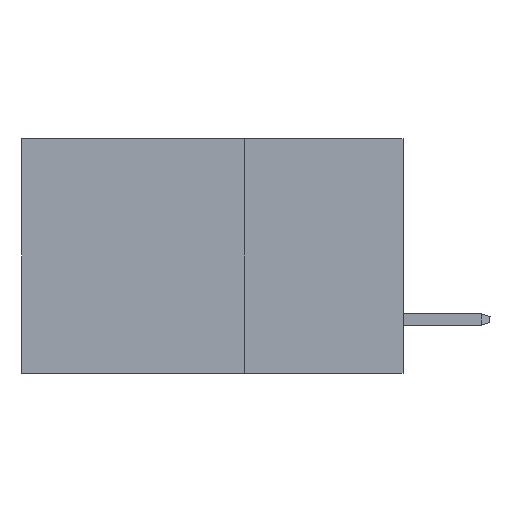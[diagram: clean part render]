
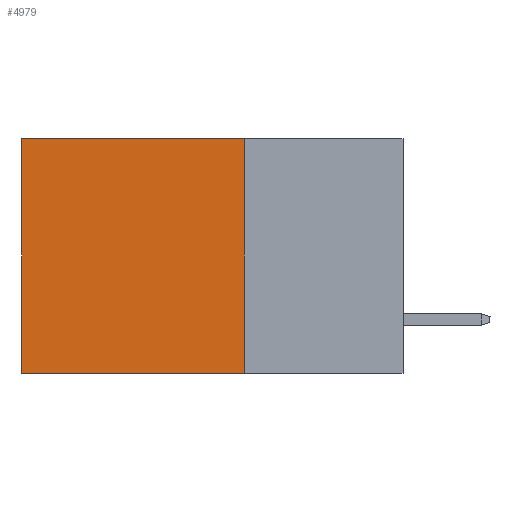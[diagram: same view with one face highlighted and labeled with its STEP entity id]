
A CAD part, left-side view. The second image highlights one B-rep face of the part: STEP entity #4979.
In plain terms, the highlighted planar face has unit normal (-1, 0, 0).
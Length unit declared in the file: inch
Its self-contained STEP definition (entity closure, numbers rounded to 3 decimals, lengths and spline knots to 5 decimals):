
#109 = VERTEX_POINT ( 'NONE', #10865 ) ;
#342 = ORIENTED_EDGE ( 'NONE', *, *, #12802, .T. ) ;
#1265 = CARTESIAN_POINT ( 'NONE',  ( 0.2875, 0.25, 0. ) ) ;
#1464 = CARTESIAN_POINT ( 'NONE',  ( 0.2875, 0.6, 0. ) ) ;
#2027 = ORIENTED_EDGE ( 'NONE', *, *, #6396, .F. ) ;
#2131 = VECTOR ( 'NONE', #9595, 39.37008 ) ;
#2871 = DIRECTION ( 'NONE',  ( 1., 0., 0. ) ) ;
#3625 = VERTEX_POINT ( 'NONE', #3956 ) ;
#3956 = CARTESIAN_POINT ( 'NONE',  ( 0.2875, 0.25, 0. ) ) ;
#4029 = FACE_OUTER_BOUND ( 'NONE', #9626, .T. ) ;
#4313 = VERTEX_POINT ( 'NONE', #4517 ) ;
#4517 = CARTESIAN_POINT ( 'NONE',  ( 0.2875, 0.6, 0. ) ) ;
#4924 = CARTESIAN_POINT ( 'NONE',  ( 0.2875, 0.25, -0.37 ) ) ;
#4979 = ADVANCED_FACE ( 'NONE', ( #4029 ), #5988, .F. ) ;
#5329 = EDGE_CURVE ( 'NONE', #4313, #109, #6518, .T. ) ;
#5395 = DIRECTION ( 'NONE',  ( 0., 0., -1. ) ) ;
#5525 = DIRECTION ( 'NONE',  ( 0., 0., -1. ) ) ;
#5896 = ORIENTED_EDGE ( 'NONE', *, *, #7676, .F. ) ;
#5988 = PLANE ( 'NONE',  #11218 ) ;
#6044 = DIRECTION ( 'NONE',  ( 0., 1., 0. ) ) ;
#6396 = EDGE_CURVE ( 'NONE', #3625, #12689, #11311, .T. ) ;
#6518 = LINE ( 'NONE', #1464, #8659 ) ;
#7627 = VECTOR ( 'NONE', #5395, 39.37008 ) ;
#7676 = EDGE_CURVE ( 'NONE', #12689, #109, #11475, .T. ) ;
#8659 = VECTOR ( 'NONE', #5525, 39.37008 ) ;
#8897 = LINE ( 'NONE', #12933, #9411 ) ;
#9043 = CARTESIAN_POINT ( 'NONE',  ( 0.2875, 0.25, 0. ) ) ;
#9113 = DIRECTION ( 'NONE',  ( 0., 0., -1. ) ) ;
#9411 = VECTOR ( 'NONE', #6044, 39.37008 ) ;
#9595 = DIRECTION ( 'NONE',  ( 0., 1., 0. ) ) ;
#9626 = EDGE_LOOP ( 'NONE', ( #10014, #5896, #2027, #342 ) ) ;
#10014 = ORIENTED_EDGE ( 'NONE', *, *, #5329, .T. ) ;
#10605 = CARTESIAN_POINT ( 'NONE',  ( 0.2875, 0.25, -0.37 ) ) ;
#10865 = CARTESIAN_POINT ( 'NONE',  ( 0.2875, 0.6, -0.37 ) ) ;
#11218 = AXIS2_PLACEMENT_3D ( 'NONE', #9043, #2871, #9113 ) ;
#11311 = LINE ( 'NONE', #1265, #7627 ) ;
#11475 = LINE ( 'NONE', #10605, #2131 ) ;
#12689 = VERTEX_POINT ( 'NONE', #4924 ) ;
#12802 = EDGE_CURVE ( 'NONE', #3625, #4313, #8897, .T. ) ;
#12933 = CARTESIAN_POINT ( 'NONE',  ( 0.2875, 0.25, 0. ) ) ;
